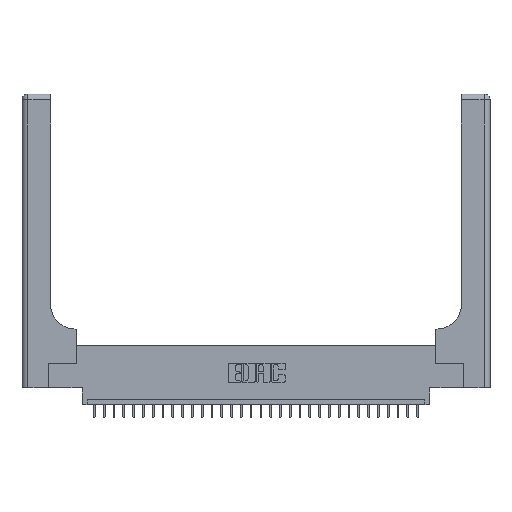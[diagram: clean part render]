
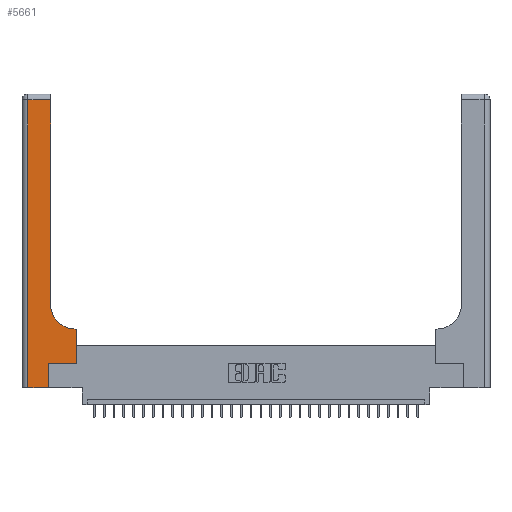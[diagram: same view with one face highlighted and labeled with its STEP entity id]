
A CAD part, top view. The second image highlights one B-rep face of the part: STEP entity #5661.
In plain terms, the highlighted planar face has unit normal (0, 0, 1).
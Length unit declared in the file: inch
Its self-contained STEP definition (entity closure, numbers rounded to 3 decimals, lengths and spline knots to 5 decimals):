
#191 = VERTEX_POINT ( 'NONE', #800 ) ;
#478 = EDGE_CURVE ( 'NONE', #8936, #28675, #19932, .T. ) ;
#800 = CARTESIAN_POINT ( 'NONE',  ( 0.06, 2.94, 0.37 ) ) ;
#1568 = LINE ( 'NONE', #23495, #18654 ) ;
#1762 = DIRECTION ( 'NONE',  ( -1., 0., 0. ) ) ;
#1781 = ORIENTED_EDGE ( 'NONE', *, *, #13900, .T. ) ;
#2211 = DIRECTION ( 'NONE',  ( 0., 1., 0. ) ) ;
#2402 = DIRECTION ( 'NONE',  ( 0., 1., 0. ) ) ;
#2664 = CIRCLE ( 'NONE', #3171, 0.25 ) ;
#2968 = VECTOR ( 'NONE', #2402, 39.37008 ) ;
#3010 = CARTESIAN_POINT ( 'NONE',  ( 0., 3., 0.37 ) ) ;
#3171 = AXIS2_PLACEMENT_3D ( 'NONE', #24394, #11585, #14024 ) ;
#3381 = VERTEX_POINT ( 'NONE', #17081 ) ;
#4809 = LINE ( 'NONE', #16526, #5705 ) ;
#4835 = CARTESIAN_POINT ( 'NONE',  ( 0.5585, 0.25, 0.37 ) ) ;
#5447 = FACE_OUTER_BOUND ( 'NONE', #26533, .T. ) ;
#5661 = ADVANCED_FACE ( 'NONE', ( #5447 ), #30250, .F. ) ;
#5705 = VECTOR ( 'NONE', #2211, 39.37008 ) ;
#5720 = VECTOR ( 'NONE', #25019, 39.37008 ) ;
#5774 = DIRECTION ( 'NONE',  ( 0., 0., -1. ) ) ;
#6111 = EDGE_CURVE ( 'NONE', #31692, #191, #24013, .T. ) ;
#6751 = CARTESIAN_POINT ( 'NONE',  ( 0.5585, 0.25, 0.37 ) ) ;
#7532 = CARTESIAN_POINT ( 'NONE',  ( 0.5415, 0.6, 0.37 ) ) ;
#7969 = EDGE_CURVE ( 'NONE', #25297, #22152, #2664, .T. ) ;
#8788 = ORIENTED_EDGE ( 'NONE', *, *, #13650, .T. ) ;
#8936 = VERTEX_POINT ( 'NONE', #6751 ) ;
#9214 = CARTESIAN_POINT ( 'NONE',  ( 0.06, 3., 0.37 ) ) ;
#9664 = ORIENTED_EDGE ( 'NONE', *, *, #27990, .T. ) ;
#9933 = LINE ( 'NONE', #15123, #5720 ) ;
#10443 = VECTOR ( 'NONE', #1762, 39.37008 ) ;
#11326 = CARTESIAN_POINT ( 'NONE',  ( 0.269, 0., 0.37 ) ) ;
#11585 = DIRECTION ( 'NONE',  ( 0., 0., -1. ) ) ;
#11909 = ORIENTED_EDGE ( 'NONE', *, *, #7969, .T. ) ;
#12506 = ORIENTED_EDGE ( 'NONE', *, *, #28476, .T. ) ;
#13650 = EDGE_CURVE ( 'NONE', #191, #23308, #19440, .T. ) ;
#13900 = EDGE_CURVE ( 'NONE', #28675, #25297, #24062, .T. ) ;
#14024 = DIRECTION ( 'NONE',  ( 1., 0., 0. ) ) ;
#15123 = CARTESIAN_POINT ( 'NONE',  ( 0., 0., 0.37 ) ) ;
#16526 = CARTESIAN_POINT ( 'NONE',  ( 0.2915, 3., 0.37 ) ) ;
#16941 = VECTOR ( 'NONE', #28831, 39.37008 ) ;
#17081 = CARTESIAN_POINT ( 'NONE',  ( 0.269, 0.25, 0.37 ) ) ;
#17638 = DIRECTION ( 'NONE',  ( -1., 0., 0. ) ) ;
#17882 = CARTESIAN_POINT ( 'NONE',  ( 0.5585, 0.6, 0.37 ) ) ;
#18317 = DIRECTION ( 'NONE',  ( 0., 1., 0. ) ) ;
#18654 = VECTOR ( 'NONE', #18317, 39.37008 ) ;
#18734 = CARTESIAN_POINT ( 'NONE',  ( 0.2915, 0.6, 0.37 ) ) ;
#19440 = LINE ( 'NONE', #9214, #16941 ) ;
#19737 = AXIS2_PLACEMENT_3D ( 'NONE', #3010, #5774, #17638 ) ;
#19932 = LINE ( 'NONE', #4835, #2968 ) ;
#22152 = VERTEX_POINT ( 'NONE', #25556 ) ;
#23308 = VERTEX_POINT ( 'NONE', #27062 ) ;
#23495 = CARTESIAN_POINT ( 'NONE',  ( 0.269, 0., 0.37 ) ) ;
#23543 = VERTEX_POINT ( 'NONE', #11326 ) ;
#24013 = LINE ( 'NONE', #26271, #10443 ) ;
#24062 = LINE ( 'NONE', #18734, #31850 ) ;
#24350 = ORIENTED_EDGE ( 'NONE', *, *, #478, .T. ) ;
#24394 = CARTESIAN_POINT ( 'NONE',  ( 0.5415, 0.85, 0.37 ) ) ;
#25019 = DIRECTION ( 'NONE',  ( 1., 0., 0. ) ) ;
#25297 = VERTEX_POINT ( 'NONE', #7532 ) ;
#25556 = CARTESIAN_POINT ( 'NONE',  ( 0.2915, 0.85, 0.37 ) ) ;
#25902 = EDGE_CURVE ( 'NONE', #22152, #31692, #4809, .T. ) ;
#25923 = VECTOR ( 'NONE', #28729, 39.37008 ) ;
#26271 = CARTESIAN_POINT ( 'NONE',  ( 0., 2.94, 0.37 ) ) ;
#26324 = DIRECTION ( 'NONE',  ( -1., 0., 0. ) ) ;
#26533 = EDGE_LOOP ( 'NONE', ( #30237, #31823, #8788, #12506, #9664, #31089, #24350, #1781, #11909 ) ) ;
#27062 = CARTESIAN_POINT ( 'NONE',  ( 0.06, 0., 0.37 ) ) ;
#27990 = EDGE_CURVE ( 'NONE', #23543, #3381, #1568, .T. ) ;
#28389 = EDGE_CURVE ( 'NONE', #3381, #8936, #31324, .T. ) ;
#28421 = CARTESIAN_POINT ( 'NONE',  ( 0.269, 0.25, 0.37 ) ) ;
#28476 = EDGE_CURVE ( 'NONE', #23308, #23543, #9933, .T. ) ;
#28675 = VERTEX_POINT ( 'NONE', #17882 ) ;
#28729 = DIRECTION ( 'NONE',  ( 1., 0., 0. ) ) ;
#28831 = DIRECTION ( 'NONE',  ( 0., -1., 0. ) ) ;
#29345 = CARTESIAN_POINT ( 'NONE',  ( 0.2915, 2.94, 0.37 ) ) ;
#30237 = ORIENTED_EDGE ( 'NONE', *, *, #25902, .T. ) ;
#30250 = PLANE ( 'NONE',  #19737 ) ;
#31089 = ORIENTED_EDGE ( 'NONE', *, *, #28389, .T. ) ;
#31324 = LINE ( 'NONE', #28421, #25923 ) ;
#31692 = VERTEX_POINT ( 'NONE', #29345 ) ;
#31823 = ORIENTED_EDGE ( 'NONE', *, *, #6111, .T. ) ;
#31850 = VECTOR ( 'NONE', #26324, 39.37008 ) ;
